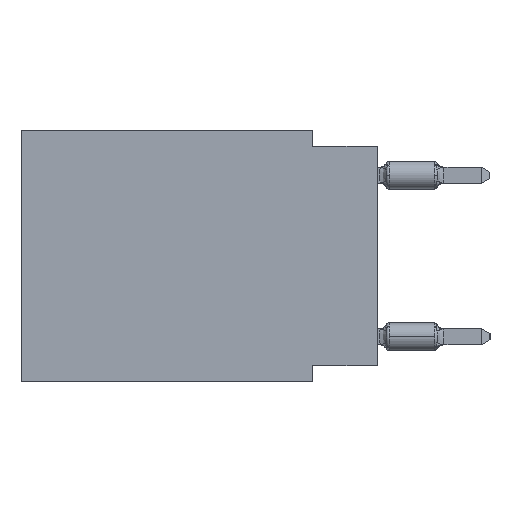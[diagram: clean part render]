
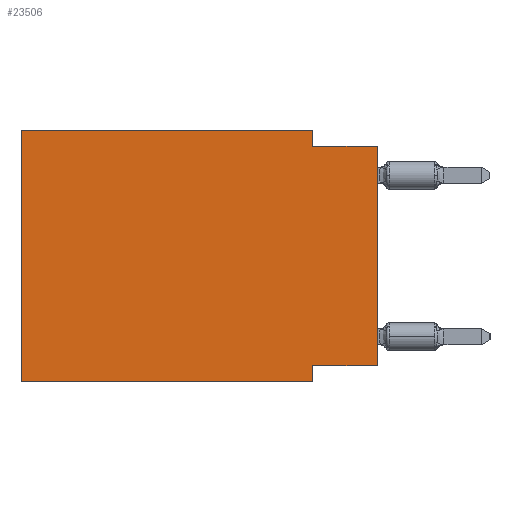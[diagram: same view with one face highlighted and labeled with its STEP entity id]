
A CAD part, left-side view. The second image highlights one B-rep face of the part: STEP entity #23506.
In plain terms, the highlighted planar face has unit normal (-1, 0, 0).
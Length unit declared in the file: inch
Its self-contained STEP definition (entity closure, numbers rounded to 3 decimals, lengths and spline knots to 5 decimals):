
#108 = LINE ( 'NONE', #4446, #13047 ) ;
#475 = CARTESIAN_POINT ( 'NONE',  ( 0., 0.1, 0. ) ) ;
#558 = ORIENTED_EDGE ( 'NONE', *, *, #25881, .F. ) ;
#745 = VECTOR ( 'NONE', #26191, 39.37008 ) ;
#1222 = VECTOR ( 'NONE', #15316, 39.37008 ) ;
#1927 = VERTEX_POINT ( 'NONE', #9655 ) ;
#2203 = VERTEX_POINT ( 'NONE', #20397 ) ;
#2403 = ORIENTED_EDGE ( 'NONE', *, *, #26482, .F. ) ;
#3423 = AXIS2_PLACEMENT_3D ( 'NONE', #4789, #5209, #13529 ) ;
#4298 = ORIENTED_EDGE ( 'NONE', *, *, #28119, .F. ) ;
#4370 = CARTESIAN_POINT ( 'NONE',  ( 0., 0.1, 0. ) ) ;
#4446 = CARTESIAN_POINT ( 'NONE',  ( 0., 0., -0.365 ) ) ;
#4648 = PLANE ( 'NONE',  #3423 ) ;
#4789 = CARTESIAN_POINT ( 'NONE',  ( 0., 0.55, 0. ) ) ;
#5045 = CARTESIAN_POINT ( 'NONE',  ( 0., 0.55, 0. ) ) ;
#5208 = LINE ( 'NONE', #5498, #24321 ) ;
#5209 = DIRECTION ( 'NONE',  ( 1., 0., 0. ) ) ;
#5498 = CARTESIAN_POINT ( 'NONE',  ( 0., 0., -0.025 ) ) ;
#6155 = CARTESIAN_POINT ( 'NONE',  ( 0., 0.1, -0.39 ) ) ;
#6477 = CARTESIAN_POINT ( 'NONE',  ( 0., 0.55, 0. ) ) ;
#7439 = DIRECTION ( 'NONE',  ( 0., 0., 1. ) ) ;
#7847 = CARTESIAN_POINT ( 'NONE',  ( 0., 0.1, -0.39 ) ) ;
#8615 = DIRECTION ( 'NONE',  ( 0., -1., 0. ) ) ;
#8965 = LINE ( 'NONE', #19728, #15928 ) ;
#9655 = CARTESIAN_POINT ( 'NONE',  ( 0., 0., -0.365 ) ) ;
#10867 = LINE ( 'NONE', #6155, #1222 ) ;
#11271 = EDGE_CURVE ( 'NONE', #24177, #20892, #5208, .T. ) ;
#11273 = CARTESIAN_POINT ( 'NONE',  ( 0., 0.1, -0.025 ) ) ;
#11638 = LINE ( 'NONE', #5045, #745 ) ;
#13047 = VECTOR ( 'NONE', #17061, 39.37008 ) ;
#13191 = ORIENTED_EDGE ( 'NONE', *, *, #11271, .F. ) ;
#13529 = DIRECTION ( 'NONE',  ( 0., 0., -1. ) ) ;
#13819 = ORIENTED_EDGE ( 'NONE', *, *, #27727, .F. ) ;
#13947 = DIRECTION ( 'NONE',  ( 0., -1., 0. ) ) ;
#15266 = DIRECTION ( 'NONE',  ( 0., 0., -1. ) ) ;
#15316 = DIRECTION ( 'NONE',  ( 0., 0., -1. ) ) ;
#15429 = VECTOR ( 'NONE', #8615, 39.37008 ) ;
#15928 = VECTOR ( 'NONE', #22308, 39.37008 ) ;
#16538 = VERTEX_POINT ( 'NONE', #23089 ) ;
#16837 = CARTESIAN_POINT ( 'NONE',  ( 0., 0.55, -0.39 ) ) ;
#17061 = DIRECTION ( 'NONE',  ( 0., 1., 0. ) ) ;
#17360 = LINE ( 'NONE', #6477, #15429 ) ;
#17443 = VERTEX_POINT ( 'NONE', #16837 ) ;
#18194 = VECTOR ( 'NONE', #7439, 39.37008 ) ;
#18335 = ORIENTED_EDGE ( 'NONE', *, *, #27393, .F. ) ;
#18508 = VERTEX_POINT ( 'NONE', #475 ) ;
#18624 = EDGE_CURVE ( 'NONE', #17443, #22897, #8965, .T. ) ;
#19728 = CARTESIAN_POINT ( 'NONE',  ( 0., 0.55, -0.39 ) ) ;
#20135 = FACE_OUTER_BOUND ( 'NONE', #25029, .T. ) ;
#20221 = LINE ( 'NONE', #27092, #18194 ) ;
#20397 = CARTESIAN_POINT ( 'NONE',  ( 0., 0.55, 0. ) ) ;
#20892 = VERTEX_POINT ( 'NONE', #27813 ) ;
#21673 = ORIENTED_EDGE ( 'NONE', *, *, #18624, .T. ) ;
#22308 = DIRECTION ( 'NONE',  ( 0., -1., 0. ) ) ;
#22628 = VECTOR ( 'NONE', #15266, 39.37008 ) ;
#22897 = VERTEX_POINT ( 'NONE', #7847 ) ;
#23089 = CARTESIAN_POINT ( 'NONE',  ( 0., 0.1, -0.365 ) ) ;
#23506 = ADVANCED_FACE ( 'NONE', ( #20135 ), #4648, .F. ) ;
#24177 = VERTEX_POINT ( 'NONE', #11273 ) ;
#24321 = VECTOR ( 'NONE', #13947, 39.37008 ) ;
#25029 = EDGE_LOOP ( 'NONE', ( #27413, #13191, #558, #13819, #18335, #21673, #4298, #2403 ) ) ;
#25881 = EDGE_CURVE ( 'NONE', #18508, #24177, #26034, .T. ) ;
#26034 = LINE ( 'NONE', #4370, #22628 ) ;
#26191 = DIRECTION ( 'NONE',  ( 0., 0., 1. ) ) ;
#26482 = EDGE_CURVE ( 'NONE', #1927, #16538, #108, .T. ) ;
#27092 = CARTESIAN_POINT ( 'NONE',  ( 0., 0., 0. ) ) ;
#27393 = EDGE_CURVE ( 'NONE', #17443, #2203, #11638, .T. ) ;
#27413 = ORIENTED_EDGE ( 'NONE', *, *, #27857, .T. ) ;
#27727 = EDGE_CURVE ( 'NONE', #2203, #18508, #17360, .T. ) ;
#27813 = CARTESIAN_POINT ( 'NONE',  ( 0., 0., -0.025 ) ) ;
#27857 = EDGE_CURVE ( 'NONE', #1927, #20892, #20221, .T. ) ;
#28119 = EDGE_CURVE ( 'NONE', #16538, #22897, #10867, .T. ) ;
